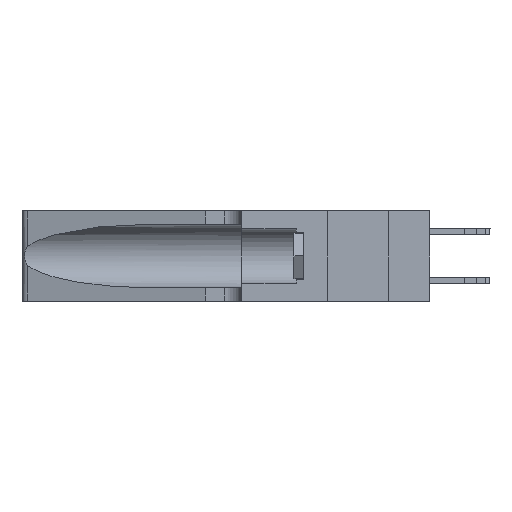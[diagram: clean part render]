
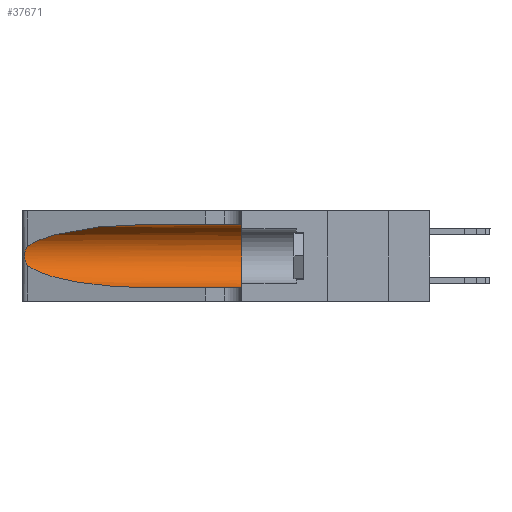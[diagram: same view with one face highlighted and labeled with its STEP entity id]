
A CAD part, left-side view. The second image highlights one B-rep face of the part: STEP entity #37671.
In plain terms, the highlighted cylindrical face has radius 3.308 mm (diameter 6.617 mm), a partial arc.
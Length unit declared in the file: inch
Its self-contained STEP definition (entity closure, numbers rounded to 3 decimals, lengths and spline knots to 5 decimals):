
#1031 = CARTESIAN_POINT ( 'NONE',  ( 0.1305, 0.35, 0.185 ) ) ;
#2424 = CARTESIAN_POINT ( 'NONE',  ( 0.1305, 0.35, 0.31525 ) ) ;
#3623 = FACE_OUTER_BOUND ( 'NONE', #20747, .T. ) ;
#3987 = CARTESIAN_POINT ( 'NONE',  ( 0.26018, 1.23835, 0.19895 ) ) ;
#3998 = CARTESIAN_POINT ( 'NONE',  ( 0.2373, 1.15595, 0.28018 ) ) ;
#4741 = VERTEX_POINT ( 'NONE', #7938 ) ;
#6481 = DIRECTION ( 'NONE',  ( 0., -1., 0. ) ) ;
#7092 = CARTESIAN_POINT ( 'NONE',  ( 0.26075, 1.23896, 0.19203 ) ) ;
#7105 = CARTESIAN_POINT ( 'NONE',  ( 0.18966, 0.96281, 0.31525 ) ) ;
#7938 = CARTESIAN_POINT ( 'NONE',  ( 0.1305, 0.35, 0.05475 ) ) ;
#9330 = AXIS2_PLACEMENT_3D ( 'NONE', #9420, #6481, #30774 ) ;
#9420 = CARTESIAN_POINT ( 'NONE',  ( 0.1305, 1.61858, 0.185 ) ) ;
#10101 = CARTESIAN_POINT ( 'NONE',  ( 0.18966, 0.96281, 0.05475 ) ) ;
#10512 = CARTESIAN_POINT ( 'NONE',  ( 0.1305, 0.72297, 0.05475 ) ) ;
#11717 = B_SPLINE_CURVE_WITH_KNOTS ( 'NONE', 3,
 ( #37697, #22401, #16087, #37567, #16618, #3987, #7092, #37825, #16353, #22830, #31395, #19201, #25381, #28463 ),
 .UNSPECIFIED., .F., .F.,
 ( 4, 2, 2, 2, 2, 2, 4 ),
 ( 0., 0.00027, 0.00053, 0.00107, 0.0016, 0.00187, 0.00214 ),
 .UNSPECIFIED. ) ;
#12152 = CIRCLE ( 'NONE', #33337, 0.13025 ) ;
#13621 = CARTESIAN_POINT ( 'NONE',  ( 0.2373, 1.15595, 0.08982 ) ) ;
#14135 = VERTEX_POINT ( 'NONE', #16238 ) ;
#15230 = ORIENTED_EDGE ( 'NONE', *, *, #39719, .F. ) ;
#15606 = CARTESIAN_POINT ( 'NONE',  ( 0.1305, 1.61858, 0.31525 ) ) ;
#16087 = CARTESIAN_POINT ( 'NONE',  ( 0.25639, 1.23184, 0.21858 ) ) ;
#16192 = ORIENTED_EDGE ( 'NONE', *, *, #17526, .T. ) ;
#16238 = CARTESIAN_POINT ( 'NONE',  ( 0.25487, 1.22718, 0.22369 ) ) ;
#16353 = CARTESIAN_POINT ( 'NONE',  ( 0.26017, 1.23833, 0.17102 ) ) ;
#16575 = ORIENTED_EDGE ( 'NONE', *, *, #33790, .T. ) ;
#16618 = CARTESIAN_POINT ( 'NONE',  ( 0.25854, 1.2359, 0.20912 ) ) ;
#16819 = ORIENTED_EDGE ( 'NONE', *, *, #31673, .T. ) ;
#17526 = EDGE_CURVE ( 'NONE', #24175, #14135, #17858, .T. ) ;
#17858 =( BOUNDED_CURVE ( )  B_SPLINE_CURVE ( 3, ( #31001, #7105, #3998, #25391 ),
 .UNSPECIFIED., .F., .F. ) 
 B_SPLINE_CURVE_WITH_KNOTS ( ( 4, 4 ),
 ( 1.5708, 2.84003 ),
 .UNSPECIFIED. ) 
 CURVE ( )  GEOMETRIC_REPRESENTATION_ITEM ( )  RATIONAL_B_SPLINE_CURVE ( ( 1., 0.87, 0.87, 1. ) ) 
 REPRESENTATION_ITEM ( '' )  );
#18740 = VERTEX_POINT ( 'NONE', #2424 ) ;
#19052 = DIRECTION ( 'NONE',  ( 0., 0., 1. ) ) ;
#19201 = CARTESIAN_POINT ( 'NONE',  ( 0.25639, 1.23186, 0.15144 ) ) ;
#19214 = CARTESIAN_POINT ( 'NONE',  ( 0.1305, 0.72297, 0.31525 ) ) ;
#20747 = EDGE_LOOP ( 'NONE', ( #16192, #26689, #16819, #16575, #15230, #34736 ) ) ;
#21793 = DIRECTION ( 'NONE',  ( 0., -1., 0. ) ) ;
#22401 = CARTESIAN_POINT ( 'NONE',  ( 0.25555, 1.22994, 0.2215 ) ) ;
#22537 = DIRECTION ( 'NONE',  ( 0., 1., 0. ) ) ;
#22830 = CARTESIAN_POINT ( 'NONE',  ( 0.25856, 1.23593, 0.16098 ) ) ;
#22960 = LINE ( 'NONE', #15606, #33941 ) ;
#23269 = DIRECTION ( 'NONE',  ( 0., -1., 0. ) ) ;
#24175 = VERTEX_POINT ( 'NONE', #19214 ) ;
#25381 = CARTESIAN_POINT ( 'NONE',  ( 0.25555, 1.22993, 0.14849 ) ) ;
#25391 = CARTESIAN_POINT ( 'NONE',  ( 0.25487, 1.22718, 0.22369 ) ) ;
#26689 = ORIENTED_EDGE ( 'NONE', *, *, #27153, .T. ) ;
#27153 = EDGE_CURVE ( 'NONE', #14135, #33186, #11717, .T. ) ;
#27933 = VERTEX_POINT ( 'NONE', #36411 ) ;
#28463 = CARTESIAN_POINT ( 'NONE',  ( 0.25487, 1.22718, 0.14631 ) ) ;
#29087 = CYLINDRICAL_SURFACE ( 'NONE', #9330, 0.13025 ) ;
#29796 = EDGE_CURVE ( 'NONE', #24175, #18740, #22960, .T. ) ;
#30774 = DIRECTION ( 'NONE',  ( 0., 0., -1. ) ) ;
#31001 = CARTESIAN_POINT ( 'NONE',  ( 0.1305, 0.72297, 0.31525 ) ) ;
#31315 = VECTOR ( 'NONE', #23269, 39.37008 ) ;
#31395 = CARTESIAN_POINT ( 'NONE',  ( 0.25789, 1.23486, 0.15765 ) ) ;
#31673 = EDGE_CURVE ( 'NONE', #33186, #27933, #34290, .T. ) ;
#32226 = CARTESIAN_POINT ( 'NONE',  ( 0.1305, 1.61858, 0.05475 ) ) ;
#33186 = VERTEX_POINT ( 'NONE', #37169 ) ;
#33337 = AXIS2_PLACEMENT_3D ( 'NONE', #1031, #22537, #19052 ) ;
#33790 = EDGE_CURVE ( 'NONE', #27933, #4741, #38526, .T. ) ;
#33941 = VECTOR ( 'NONE', #21793, 39.37008 ) ;
#34290 =( BOUNDED_CURVE ( )  B_SPLINE_CURVE ( 3, ( #35176, #13621, #10101, #10512 ),
 .UNSPECIFIED., .F., .F. ) 
 B_SPLINE_CURVE_WITH_KNOTS ( ( 4, 4 ),
 ( 3.44316, 4.71239 ),
 .UNSPECIFIED. ) 
 CURVE ( )  GEOMETRIC_REPRESENTATION_ITEM ( )  RATIONAL_B_SPLINE_CURVE ( ( 1., 0.87, 0.87, 1. ) ) 
 REPRESENTATION_ITEM ( '' )  );
#34736 = ORIENTED_EDGE ( 'NONE', *, *, #29796, .F. ) ;
#35176 = CARTESIAN_POINT ( 'NONE',  ( 0.25487, 1.22718, 0.14631 ) ) ;
#36411 = CARTESIAN_POINT ( 'NONE',  ( 0.1305, 0.72297, 0.05475 ) ) ;
#37169 = CARTESIAN_POINT ( 'NONE',  ( 0.25487, 1.22718, 0.14631 ) ) ;
#37567 = CARTESIAN_POINT ( 'NONE',  ( 0.25787, 1.23484, 0.2124 ) ) ;
#37671 = ADVANCED_FACE ( 'NONE', ( #3623 ), #29087, .F. ) ;
#37697 = CARTESIAN_POINT ( 'NONE',  ( 0.25487, 1.22718, 0.22369 ) ) ;
#37825 = CARTESIAN_POINT ( 'NONE',  ( 0.26075, 1.23896, 0.178 ) ) ;
#38526 = LINE ( 'NONE', #32226, #31315 ) ;
#39719 = EDGE_CURVE ( 'NONE', #18740, #4741, #12152, .T. ) ;
